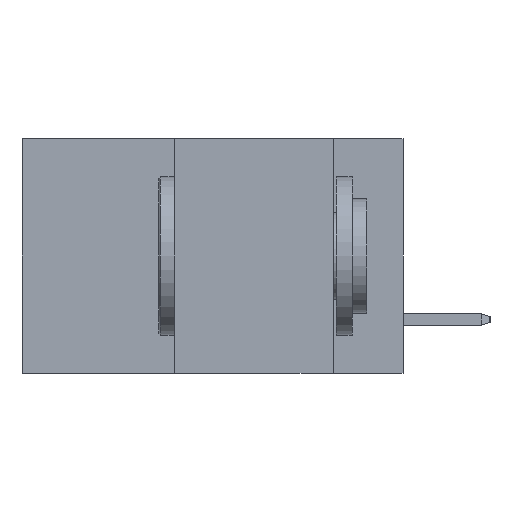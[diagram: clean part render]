
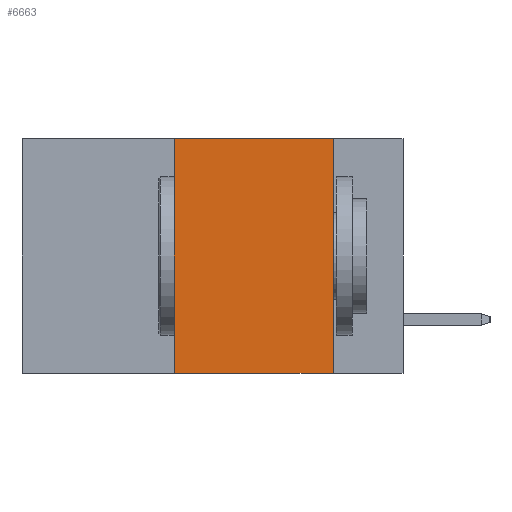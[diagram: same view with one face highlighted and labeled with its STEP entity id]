
A CAD part, left-side view. The second image highlights one B-rep face of the part: STEP entity #6663.
In plain terms, the highlighted planar face has unit normal (-1, 0, 0).
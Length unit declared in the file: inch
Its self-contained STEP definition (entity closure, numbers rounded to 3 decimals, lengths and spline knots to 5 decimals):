
#353 = FACE_OUTER_BOUND ( 'NONE', #5929, .T. ) ;
#407 = DIRECTION ( 'NONE',  ( 1., 0., 0. ) ) ;
#435 = EDGE_CURVE ( 'NONE', #2796, #9357, #2892, .T. ) ;
#600 = EDGE_CURVE ( 'NONE', #2476, #9357, #3826, .T. ) ;
#1095 = VECTOR ( 'NONE', #6419, 39.37008 ) ;
#1202 = CARTESIAN_POINT ( 'NONE',  ( 0., 0.11, -0.37 ) ) ;
#1982 = CARTESIAN_POINT ( 'NONE',  ( 0., 0.36, 0. ) ) ;
#2466 = CARTESIAN_POINT ( 'NONE',  ( 0., 0.11, 0. ) ) ;
#2476 = VERTEX_POINT ( 'NONE', #2466 ) ;
#2496 = CARTESIAN_POINT ( 'NONE',  ( 0., 0.36, -0.37 ) ) ;
#2796 = VERTEX_POINT ( 'NONE', #2496 ) ;
#2838 = DIRECTION ( 'NONE',  ( 0., -1., 0. ) ) ;
#2892 = LINE ( 'NONE', #4359, #8072 ) ;
#2983 = EDGE_CURVE ( 'NONE', #7726, #2476, #7878, .T. ) ;
#3322 = ORIENTED_EDGE ( 'NONE', *, *, #2983, .F. ) ;
#3777 = DIRECTION ( 'NONE',  ( 0., 0., 1. ) ) ;
#3826 = LINE ( 'NONE', #9610, #5280 ) ;
#4130 = ORIENTED_EDGE ( 'NONE', *, *, #435, .T. ) ;
#4235 = CARTESIAN_POINT ( 'NONE',  ( 0., 0.6, 0. ) ) ;
#4359 = CARTESIAN_POINT ( 'NONE',  ( 0., 0.6, -0.37 ) ) ;
#4870 = CARTESIAN_POINT ( 'NONE',  ( 0., 0.6, 0. ) ) ;
#4893 = AXIS2_PLACEMENT_3D ( 'NONE', #4870, #407, #9260 ) ;
#5092 = LINE ( 'NONE', #8100, #9554 ) ;
#5176 = ORIENTED_EDGE ( 'NONE', *, *, #600, .F. ) ;
#5236 = DIRECTION ( 'NONE',  ( 0., 0., -1. ) ) ;
#5280 = VECTOR ( 'NONE', #5236, 39.37008 ) ;
#5331 = PLANE ( 'NONE',  #4893 ) ;
#5929 = EDGE_LOOP ( 'NONE', ( #5176, #3322, #8315, #4130 ) ) ;
#6419 = DIRECTION ( 'NONE',  ( 0., -1., 0. ) ) ;
#6472 = EDGE_CURVE ( 'NONE', #2796, #7726, #5092, .T. ) ;
#6663 = ADVANCED_FACE ( 'NONE', ( #353 ), #5331, .F. ) ;
#7726 = VERTEX_POINT ( 'NONE', #1982 ) ;
#7878 = LINE ( 'NONE', #4235, #1095 ) ;
#8072 = VECTOR ( 'NONE', #2838, 39.37008 ) ;
#8100 = CARTESIAN_POINT ( 'NONE',  ( 0., 0.36, 0. ) ) ;
#8315 = ORIENTED_EDGE ( 'NONE', *, *, #6472, .F. ) ;
#9260 = DIRECTION ( 'NONE',  ( 0., 0., -1. ) ) ;
#9357 = VERTEX_POINT ( 'NONE', #1202 ) ;
#9554 = VECTOR ( 'NONE', #3777, 39.37008 ) ;
#9610 = CARTESIAN_POINT ( 'NONE',  ( 0., 0.11, 0. ) ) ;
